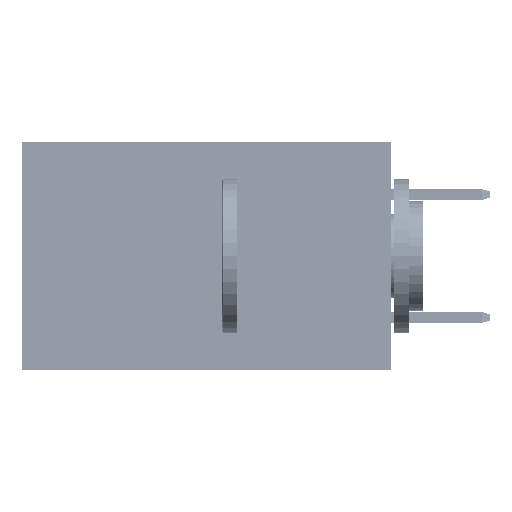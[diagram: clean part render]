
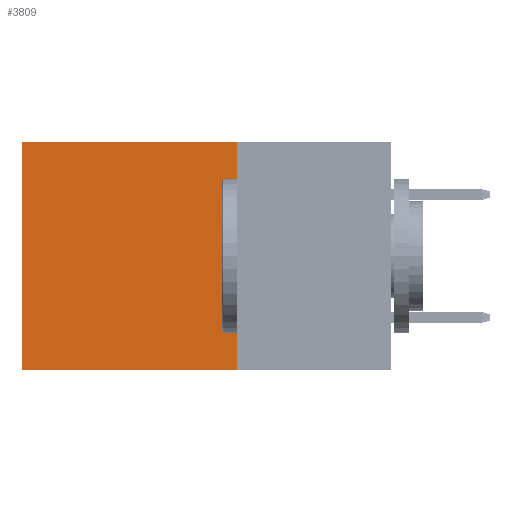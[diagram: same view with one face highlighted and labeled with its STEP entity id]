
A CAD part, left-side view. The second image highlights one B-rep face of the part: STEP entity #3809.
In plain terms, the highlighted planar face has unit normal (-1, 0, 0).
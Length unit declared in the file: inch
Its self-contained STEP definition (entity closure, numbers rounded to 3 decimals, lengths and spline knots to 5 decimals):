
#787 = CARTESIAN_POINT ( 'NONE',  ( 0.2875, 0.6, -0.37 ) ) ;
#799 = DIRECTION ( 'NONE',  ( 1., 0., 0. ) ) ;
#1075 = EDGE_LOOP ( 'NONE', ( #25979, #43250, #3279, #9918 ) ) ;
#3279 = ORIENTED_EDGE ( 'NONE', *, *, #21468, .F. ) ;
#3809 = ADVANCED_FACE ( 'NONE', ( #44297 ), #4566, .F. ) ;
#4296 = VECTOR ( 'NONE', #44810, 39.37008 ) ;
#4566 = PLANE ( 'NONE',  #46369 ) ;
#6986 = CARTESIAN_POINT ( 'NONE',  ( 0.2875, 0.25, -0.37 ) ) ;
#7080 = EDGE_CURVE ( 'NONE', #17715, #22965, #9970, .T. ) ;
#7810 = CARTESIAN_POINT ( 'NONE',  ( 0.2875, 0.25, 0. ) ) ;
#8491 = DIRECTION ( 'NONE',  ( 0., 0., -1. ) ) ;
#9458 = DIRECTION ( 'NONE',  ( 0., 1., 0. ) ) ;
#9918 = ORIENTED_EDGE ( 'NONE', *, *, #18735, .T. ) ;
#9970 = LINE ( 'NONE', #38269, #39315 ) ;
#13397 = CARTESIAN_POINT ( 'NONE',  ( 0.2875, 0.25, -0.37 ) ) ;
#14315 = LINE ( 'NONE', #45932, #18032 ) ;
#15315 = LINE ( 'NONE', #44471, #4296 ) ;
#17715 = VERTEX_POINT ( 'NONE', #21123 ) ;
#18032 = VECTOR ( 'NONE', #22560, 39.37008 ) ;
#18735 = EDGE_CURVE ( 'NONE', #19751, #17715, #14315, .T. ) ;
#19751 = VERTEX_POINT ( 'NONE', #35074 ) ;
#21123 = CARTESIAN_POINT ( 'NONE',  ( 0.2875, 0.6, 0. ) ) ;
#21468 = EDGE_CURVE ( 'NONE', #19751, #32721, #15315, .T. ) ;
#22560 = DIRECTION ( 'NONE',  ( 0., 1., 0. ) ) ;
#22965 = VERTEX_POINT ( 'NONE', #787 ) ;
#25979 = ORIENTED_EDGE ( 'NONE', *, *, #7080, .T. ) ;
#30706 = LINE ( 'NONE', #13397, #39209 ) ;
#32721 = VERTEX_POINT ( 'NONE', #6986 ) ;
#35074 = CARTESIAN_POINT ( 'NONE',  ( 0.2875, 0.25, 0. ) ) ;
#37785 = DIRECTION ( 'NONE',  ( 0., 0., -1. ) ) ;
#38269 = CARTESIAN_POINT ( 'NONE',  ( 0.2875, 0.6, 0. ) ) ;
#39209 = VECTOR ( 'NONE', #9458, 39.37008 ) ;
#39315 = VECTOR ( 'NONE', #37785, 39.37008 ) ;
#43250 = ORIENTED_EDGE ( 'NONE', *, *, #44286, .F. ) ;
#44286 = EDGE_CURVE ( 'NONE', #32721, #22965, #30706, .T. ) ;
#44297 = FACE_OUTER_BOUND ( 'NONE', #1075, .T. ) ;
#44471 = CARTESIAN_POINT ( 'NONE',  ( 0.2875, 0.25, 0. ) ) ;
#44810 = DIRECTION ( 'NONE',  ( 0., 0., -1. ) ) ;
#45932 = CARTESIAN_POINT ( 'NONE',  ( 0.2875, 0.25, 0. ) ) ;
#46369 = AXIS2_PLACEMENT_3D ( 'NONE', #7810, #799, #8491 ) ;
